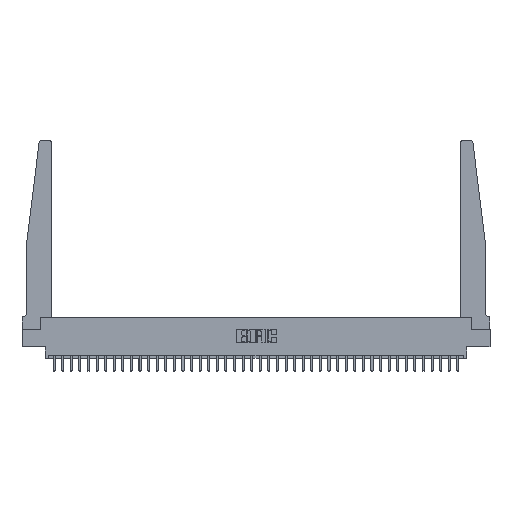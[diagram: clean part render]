
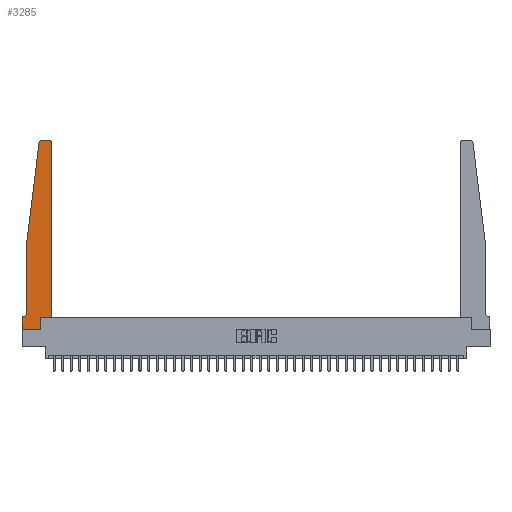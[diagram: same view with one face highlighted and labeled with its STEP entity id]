
A CAD part, top view. The second image highlights one B-rep face of the part: STEP entity #3285.
In plain terms, the highlighted planar face has unit normal (0, 0, 1).
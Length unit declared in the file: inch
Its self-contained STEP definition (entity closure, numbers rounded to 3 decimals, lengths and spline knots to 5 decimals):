
#451 = CIRCLE ( 'NONE', #7737, 0.05 ) ;
#1726 = EDGE_CURVE ( 'NONE', #2633, #16535, #11084, .T. ) ;
#1941 = CARTESIAN_POINT ( 'NONE',  ( 0.395, 2.72, 0.37 ) ) ;
#2074 = DIRECTION ( 'NONE',  ( 0., -1., 0. ) ) ;
#2165 = CARTESIAN_POINT ( 'NONE',  ( 0., 0.1875, 0.37 ) ) ;
#2633 = VERTEX_POINT ( 'NONE', #16084 ) ;
#2649 = CARTESIAN_POINT ( 'NONE',  ( 0.065, 0.1875, 0.37 ) ) ;
#2783 = VECTOR ( 'NONE', #11545, 39.37008 ) ;
#2981 = ORIENTED_EDGE ( 'NONE', *, *, #15882, .T. ) ;
#3285 = ADVANCED_FACE ( 'NONE', ( #27354 ), #35062, .T. ) ;
#3603 = DIRECTION ( 'NONE',  ( -1., 0., 0. ) ) ;
#3995 = VECTOR ( 'NONE', #5463, 39.37008 ) ;
#4064 = DIRECTION ( 'NONE',  ( 0., 1., 0. ) ) ;
#4147 = CARTESIAN_POINT ( 'NONE',  ( 0.425, 0.18, 0.37 ) ) ;
#4205 = EDGE_CURVE ( 'NONE', #20310, #11848, #451, .T. ) ;
#4336 = ORIENTED_EDGE ( 'NONE', *, *, #4205, .T. ) ;
#4779 = DIRECTION ( 'NONE',  ( 1., 0., 0. ) ) ;
#5008 = DIRECTION ( 'NONE',  ( 0., 0., 1. ) ) ;
#5220 = ORIENTED_EDGE ( 'NONE', *, *, #22333, .T. ) ;
#5463 = DIRECTION ( 'NONE',  ( -1., 0., 0. ) ) ;
#5604 = ORIENTED_EDGE ( 'NONE', *, *, #8161, .T. ) ;
#5791 = AXIS2_PLACEMENT_3D ( 'NONE', #1941, #21399, #4779 ) ;
#6977 = DIRECTION ( 'NONE',  ( 1., 0., 0. ) ) ;
#7737 = AXIS2_PLACEMENT_3D ( 'NONE', #27617, #11149, #30369 ) ;
#8155 = CARTESIAN_POINT ( 'NONE',  ( 0.2605, 0., 0.37 ) ) ;
#8161 = EDGE_CURVE ( 'NONE', #21457, #2633, #18863, .T. ) ;
#8423 = EDGE_CURVE ( 'NONE', #11192, #13147, #32890, .T. ) ;
#9103 = AXIS2_PLACEMENT_3D ( 'NONE', #2165, #5008, #24357 ) ;
#9552 = CARTESIAN_POINT ( 'NONE',  ( 0.065, 1.25, 0.37 ) ) ;
#9940 = CARTESIAN_POINT ( 'NONE',  ( 0.425, 0.18, 0.37 ) ) ;
#10037 = CARTESIAN_POINT ( 'NONE',  ( 0.2605, 0.18, 0.37 ) ) ;
#10171 = CARTESIAN_POINT ( 'NONE',  ( 0., 0., 0.37 ) ) ;
#10572 = CARTESIAN_POINT ( 'NONE',  ( 0.065, 0.2375, 0.37 ) ) ;
#11084 = LINE ( 'NONE', #19870, #2783 ) ;
#11149 = DIRECTION ( 'NONE',  ( 0., 0., -1. ) ) ;
#11192 = VERTEX_POINT ( 'NONE', #21512 ) ;
#11545 = DIRECTION ( 'NONE',  ( 1., 0., 0. ) ) ;
#11775 = ORIENTED_EDGE ( 'NONE', *, *, #26769, .T. ) ;
#11848 = VERTEX_POINT ( 'NONE', #21228 ) ;
#11968 = CARTESIAN_POINT ( 'NONE',  ( 0., 0.1875, 0.37 ) ) ;
#11980 = VERTEX_POINT ( 'NONE', #16126 ) ;
#12243 = EDGE_CURVE ( 'NONE', #24287, #11192, #13367, .T. ) ;
#13147 = VERTEX_POINT ( 'NONE', #20377 ) ;
#13367 = LINE ( 'NONE', #20219, #29715 ) ;
#13374 = CARTESIAN_POINT ( 'NONE',  ( 0.065, 1.25, 0.37 ) ) ;
#13829 = ORIENTED_EDGE ( 'NONE', *, *, #1726, .T. ) ;
#14142 = DIRECTION ( 'NONE',  ( 0., 0., 1. ) ) ;
#14355 = VECTOR ( 'NONE', #6977, 39.37008 ) ;
#14398 = CARTESIAN_POINT ( 'NONE',  ( 0.425, 2.72, 0.37 ) ) ;
#14676 = LINE ( 'NONE', #13374, #27576 ) ;
#15073 = ORIENTED_EDGE ( 'NONE', *, *, #31666, .T. ) ;
#15229 = LINE ( 'NONE', #4147, #14355 ) ;
#15653 = ORIENTED_EDGE ( 'NONE', *, *, #32221, .T. ) ;
#15882 = EDGE_CURVE ( 'NONE', #31563, #20310, #21785, .T. ) ;
#15972 = CIRCLE ( 'NONE', #5791, 0.03 ) ;
#16084 = CARTESIAN_POINT ( 'NONE',  ( 0., 0., 0.37 ) ) ;
#16126 = CARTESIAN_POINT ( 'NONE',  ( 0.2605, 0.18, 0.37 ) ) ;
#16535 = VERTEX_POINT ( 'NONE', #8155 ) ;
#17017 = VECTOR ( 'NONE', #31987, 39.37008 ) ;
#17999 = VECTOR ( 'NONE', #32100, 39.37008 ) ;
#18863 = LINE ( 'NONE', #10171, #17999 ) ;
#19870 = CARTESIAN_POINT ( 'NONE',  ( 0., 0., 0.37 ) ) ;
#20219 = CARTESIAN_POINT ( 'NONE',  ( 0.25, 2.75, 0.37 ) ) ;
#20310 = VERTEX_POINT ( 'NONE', #10572 ) ;
#20377 = CARTESIAN_POINT ( 'NONE',  ( 0.24675, 2.72367, 0.37 ) ) ;
#20796 = CARTESIAN_POINT ( 'NONE',  ( 0.425, 0.18, 0.37 ) ) ;
#21228 = CARTESIAN_POINT ( 'NONE',  ( 0.015, 0.1875, 0.37 ) ) ;
#21399 = DIRECTION ( 'NONE',  ( 0., 0., 1. ) ) ;
#21457 = VERTEX_POINT ( 'NONE', #11968 ) ;
#21512 = CARTESIAN_POINT ( 'NONE',  ( 0.27653, 2.75, 0.37 ) ) ;
#21785 = LINE ( 'NONE', #32314, #28167 ) ;
#22333 = EDGE_CURVE ( 'NONE', #11848, #21457, #26046, .T. ) ;
#22386 = AXIS2_PLACEMENT_3D ( 'NONE', #30569, #14142, #33218 ) ;
#22727 = VERTEX_POINT ( 'NONE', #9940 ) ;
#23474 = EDGE_CURVE ( 'NONE', #24654, #24287, #15972, .T. ) ;
#24287 = VERTEX_POINT ( 'NONE', #29452 ) ;
#24357 = DIRECTION ( 'NONE',  ( 1., 0., 0. ) ) ;
#24654 = VERTEX_POINT ( 'NONE', #14398 ) ;
#25173 = LINE ( 'NONE', #10037, #17017 ) ;
#25491 = ORIENTED_EDGE ( 'NONE', *, *, #23474, .T. ) ;
#26046 = LINE ( 'NONE', #2649, #3995 ) ;
#26769 = EDGE_CURVE ( 'NONE', #22727, #24654, #35299, .T. ) ;
#27319 = VECTOR ( 'NONE', #4064, 39.37008 ) ;
#27354 = FACE_OUTER_BOUND ( 'NONE', #35274, .T. ) ;
#27576 = VECTOR ( 'NONE', #35184, 39.37008 ) ;
#27617 = CARTESIAN_POINT ( 'NONE',  ( 0.015, 0.2375, 0.37 ) ) ;
#28167 = VECTOR ( 'NONE', #2074, 39.37008 ) ;
#29452 = CARTESIAN_POINT ( 'NONE',  ( 0.395, 2.75, 0.37 ) ) ;
#29715 = VECTOR ( 'NONE', #3603, 39.37008 ) ;
#30369 = DIRECTION ( 'NONE',  ( -1., 0., 0. ) ) ;
#30569 = CARTESIAN_POINT ( 'NONE',  ( 0.27653, 2.72, 0.37 ) ) ;
#31563 = VERTEX_POINT ( 'NONE', #9552 ) ;
#31666 = EDGE_CURVE ( 'NONE', #16535, #11980, #25173, .T. ) ;
#31987 = DIRECTION ( 'NONE',  ( 0., 1., 0. ) ) ;
#32100 = DIRECTION ( 'NONE',  ( 0., -1., 0. ) ) ;
#32221 = EDGE_CURVE ( 'NONE', #11980, #22727, #15229, .T. ) ;
#32314 = CARTESIAN_POINT ( 'NONE',  ( 0.065, 1.25, 0.37 ) ) ;
#32890 = CIRCLE ( 'NONE', #22386, 0.03 ) ;
#33218 = DIRECTION ( 'NONE',  ( 1., 0., 0. ) ) ;
#33365 = ORIENTED_EDGE ( 'NONE', *, *, #12243, .T. ) ;
#33813 = EDGE_CURVE ( 'NONE', #13147, #31563, #14676, .T. ) ;
#34089 = ORIENTED_EDGE ( 'NONE', *, *, #8423, .T. ) ;
#34866 = ORIENTED_EDGE ( 'NONE', *, *, #33813, .T. ) ;
#35062 = PLANE ( 'NONE',  #9103 ) ;
#35184 = DIRECTION ( 'NONE',  ( -0.122, -0.992, 0. ) ) ;
#35274 = EDGE_LOOP ( 'NONE', ( #33365, #34089, #34866, #2981, #4336, #5220, #5604, #13829, #15073, #15653, #11775, #25491 ) ) ;
#35299 = LINE ( 'NONE', #20796, #27319 ) ;
